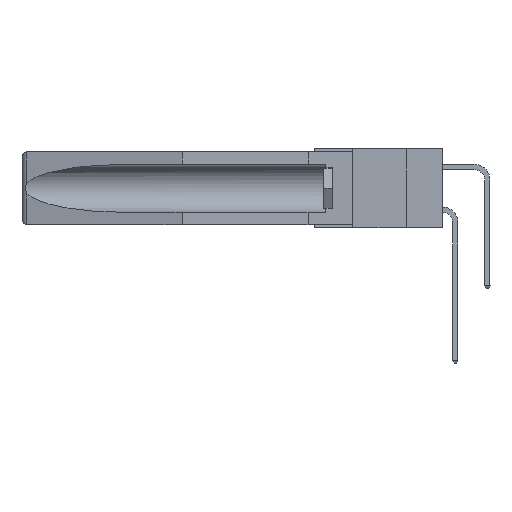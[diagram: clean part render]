
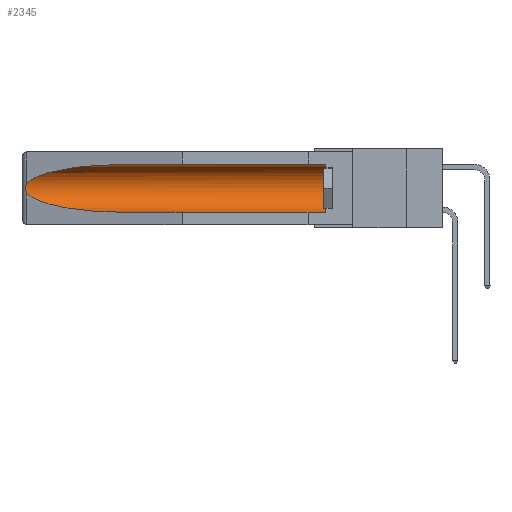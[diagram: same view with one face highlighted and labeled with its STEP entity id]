
A CAD part, left-side view. The second image highlights one B-rep face of the part: STEP entity #2345.
In plain terms, the highlighted cylindrical face has radius 2.857 mm (diameter 5.715 mm), a partial arc.
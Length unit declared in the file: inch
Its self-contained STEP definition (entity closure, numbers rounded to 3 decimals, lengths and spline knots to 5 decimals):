
#323 = AXIS2_PLACEMENT_3D ( 'NONE', #17459, #11292, #9671 ) ;
#386 = VECTOR ( 'NONE', #4373, 39.37008 ) ;
#540 = CARTESIAN_POINT ( 'NONE',  ( 0.155, 1.07973, -0.284 ) ) ;
#653 = CARTESIAN_POINT ( 'NONE',  ( 0.26537, 1.52718, -0.14972 ) ) ;
#1091 = ORIENTED_EDGE ( 'NONE', *, *, #6929, .T. ) ;
#1185 = CARTESIAN_POINT ( 'NONE',  ( 0.155, -0.30754, -0.059 ) ) ;
#1346 = AXIS2_PLACEMENT_3D ( 'NONE', #18982, #6728, #9562 ) ;
#1362 = VECTOR ( 'NONE', #7118, 39.37008 ) ;
#2023 = CARTESIAN_POINT ( 'NONE',  ( 0.26655, 1.53094, -0.18657 ) ) ;
#2101 = EDGE_CURVE ( 'NONE', #6336, #3538, #12029, .T. ) ;
#2345 = ADVANCED_FACE ( 'NONE', ( #12269 ), #16422, .F. ) ;
#2959 = CARTESIAN_POINT ( 'NONE',  ( 0.155, 1.07973, -0.059 ) ) ;
#3383 = VERTEX_POINT ( 'NONE', #2959 ) ;
#3447 = CARTESIAN_POINT ( 'NONE',  ( 0.26537, 1.52718, -0.19328 ) ) ;
#3486 = ORIENTED_EDGE ( 'NONE', *, *, #16600, .T. ) ;
#3538 = VERTEX_POINT ( 'NONE', #17259 ) ;
#4059 = CARTESIAN_POINT ( 'NONE',  ( 0.155, -0.30754, -0.284 ) ) ;
#4131 = CARTESIAN_POINT ( 'NONE',  ( 0.26537, 1.52718, -0.14972 ) ) ;
#4373 = DIRECTION ( 'NONE',  ( 0., 1., 0. ) ) ;
#4532 = ORIENTED_EDGE ( 'NONE', *, *, #11322, .F. ) ;
#5028 = CARTESIAN_POINT ( 'NONE',  ( 0.21114, 1.30732, -0.059 ) ) ;
#5088 = CARTESIAN_POINT ( 'NONE',  ( 0.2673, 1.53269, -0.17917 ) ) ;
#5295 = CARTESIAN_POINT ( 'NONE',  ( 0.25451, 1.48313, -0.24835 ) ) ;
#5648 = B_SPLINE_CURVE_WITH_KNOTS ( 'NONE', 3,
 ( #653, #14434, #19245, #6857, #11534, #9830, #5088, #2023, #17764, #14498 ),
 .UNSPECIFIED., .F., .F.,
 ( 4, 2, 2, 2, 4 ),
 ( 0., 0.00029, 0.00058, 0.00087, 0.00117 ),
 .UNSPECIFIED. ) ;
#6336 = VERTEX_POINT ( 'NONE', #11517 ) ;
#6543 = VERTEX_POINT ( 'NONE', #16045 ) ;
#6728 = DIRECTION ( 'NONE',  ( 0., 1., 0. ) ) ;
#6857 = CARTESIAN_POINT ( 'NONE',  ( 0.2673, 1.5327, -0.16383 ) ) ;
#6929 = EDGE_CURVE ( 'NONE', #3383, #11315, #17398, .T. ) ;
#7118 = DIRECTION ( 'NONE',  ( 0., 1., 0. ) ) ;
#7151 =( BOUNDED_CURVE ( )  B_SPLINE_CURVE ( 3, ( #17710, #5295, #8448, #540 ),
 .UNSPECIFIED., .F., .T. ) 
 B_SPLINE_CURVE_WITH_KNOTS ( ( 4, 4 ),
 ( 0.1948, 1.5708 ),
 .UNSPECIFIED. ) 
 CURVE ( )  GEOMETRIC_REPRESENTATION_ITEM ( )  RATIONAL_B_SPLINE_CURVE ( ( 1., 0.848, 0.848, 1. ) ) 
 REPRESENTATION_ITEM ( '' )  );
#7695 = LINE ( 'NONE', #1185, #386 ) ;
#7840 = CARTESIAN_POINT ( 'NONE',  ( 0.155, 1.07973, -0.059 ) ) ;
#8001 = EDGE_CURVE ( 'NONE', #11315, #15120, #5648, .T. ) ;
#8448 = CARTESIAN_POINT ( 'NONE',  ( 0.21114, 1.30732, -0.284 ) ) ;
#9562 = DIRECTION ( 'NONE',  ( 0., 0., 1. ) ) ;
#9671 = DIRECTION ( 'NONE',  ( 0., 0., 1. ) ) ;
#9830 = CARTESIAN_POINT ( 'NONE',  ( 0.2675, 1.53308, -0.17534 ) ) ;
#11292 = DIRECTION ( 'NONE',  ( 0., -1., 0. ) ) ;
#11315 = VERTEX_POINT ( 'NONE', #4131 ) ;
#11322 = EDGE_CURVE ( 'NONE', #6336, #6543, #11585, .T. ) ;
#11492 = EDGE_CURVE ( 'NONE', #3538, #3383, #7695, .T. ) ;
#11517 = CARTESIAN_POINT ( 'NONE',  ( 0.155, 0.126, -0.284 ) ) ;
#11534 = CARTESIAN_POINT ( 'NONE',  ( 0.2675, 1.53308, -0.16763 ) ) ;
#11585 = LINE ( 'NONE', #4059, #1362 ) ;
#12029 = CIRCLE ( 'NONE', #323, 0.1125 ) ;
#12269 = FACE_OUTER_BOUND ( 'NONE', #13247, .T. ) ;
#13247 = EDGE_LOOP ( 'NONE', ( #1091, #15770, #3486, #4532, #15589, #19800 ) ) ;
#14434 = CARTESIAN_POINT ( 'NONE',  ( 0.26597, 1.52961, -0.15275 ) ) ;
#14498 = CARTESIAN_POINT ( 'NONE',  ( 0.26537, 1.52718, -0.19328 ) ) ;
#15120 = VERTEX_POINT ( 'NONE', #3447 ) ;
#15589 = ORIENTED_EDGE ( 'NONE', *, *, #2101, .T. ) ;
#15770 = ORIENTED_EDGE ( 'NONE', *, *, #8001, .T. ) ;
#15869 = CARTESIAN_POINT ( 'NONE',  ( 0.25451, 1.48313, -0.09465 ) ) ;
#15932 = CARTESIAN_POINT ( 'NONE',  ( 0.26537, 1.52718, -0.14972 ) ) ;
#16045 = CARTESIAN_POINT ( 'NONE',  ( 0.155, 1.07973, -0.284 ) ) ;
#16422 = CYLINDRICAL_SURFACE ( 'NONE', #1346, 0.1125 ) ;
#16600 = EDGE_CURVE ( 'NONE', #15120, #6543, #7151, .T. ) ;
#17259 = CARTESIAN_POINT ( 'NONE',  ( 0.155, 0.126, -0.059 ) ) ;
#17398 =( BOUNDED_CURVE ( )  B_SPLINE_CURVE ( 3, ( #7840, #5028, #15869, #15932 ),
 .UNSPECIFIED., .F., .F. ) 
 B_SPLINE_CURVE_WITH_KNOTS ( ( 4, 4 ),
 ( 4.71239, 6.08839 ),
 .UNSPECIFIED. ) 
 CURVE ( )  GEOMETRIC_REPRESENTATION_ITEM ( )  RATIONAL_B_SPLINE_CURVE ( ( 1., 0.848, 0.848, 1. ) ) 
 REPRESENTATION_ITEM ( '' )  );
#17459 = CARTESIAN_POINT ( 'NONE',  ( 0.155, 0.126, -0.1715 ) ) ;
#17710 = CARTESIAN_POINT ( 'NONE',  ( 0.26537, 1.52718, -0.19328 ) ) ;
#17764 = CARTESIAN_POINT ( 'NONE',  ( 0.26597, 1.5296, -0.19026 ) ) ;
#18982 = CARTESIAN_POINT ( 'NONE',  ( 0.155, -0.30754, -0.1715 ) ) ;
#19245 = CARTESIAN_POINT ( 'NONE',  ( 0.26654, 1.53092, -0.15636 ) ) ;
#19800 = ORIENTED_EDGE ( 'NONE', *, *, #11492, .T. ) ;
